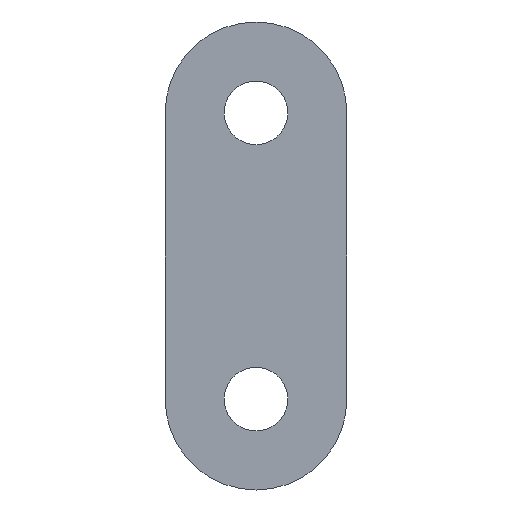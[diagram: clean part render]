
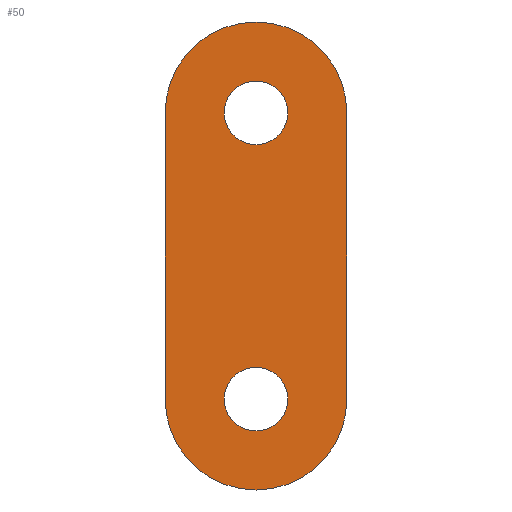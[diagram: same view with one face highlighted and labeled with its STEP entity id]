
A CAD part, left-side view. The second image highlights one B-rep face of the part: STEP entity #50.
In plain terms, the highlighted planar face has unit normal (-1, 0, 0).
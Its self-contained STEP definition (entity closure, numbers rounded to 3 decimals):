
#2 = FACE_BOUND ( 'NONE', #23, .T. ) ;
#6 = EDGE_CURVE ( 'NONE', #173, #401, #378, .T. ) ;
#10 = LINE ( 'NONE', #126, #251 ) ;
#13 = CIRCLE ( 'NONE', #390, 1.05 ) ;
#19 = ORIENTED_EDGE ( 'NONE', *, *, #31, .F. ) ;
#21 = DIRECTION ( 'NONE',  ( 0., 0., -1. ) ) ;
#22 = ORIENTED_EDGE ( 'NONE', *, *, #41, .F. ) ;
#23 = EDGE_LOOP ( 'NONE', ( #216, #328 ) ) ;
#30 = VERTEX_POINT ( 'NONE', #389 ) ;
#31 = EDGE_CURVE ( 'NONE', #175, #66, #322, .T. ) ;
#41 = EDGE_CURVE ( 'NONE', #116, #319, #157, .T. ) ;
#49 = EDGE_LOOP ( 'NONE', ( #407, #62 ) ) ;
#50 = ADVANCED_FACE ( 'NONE', ( #2, #203, #423 ), #230, .F. ) ;
#55 = ORIENTED_EDGE ( 'NONE', *, *, #72, .T. ) ;
#61 = EDGE_CURVE ( 'NONE', #319, #175, #166, .T. ) ;
#62 = ORIENTED_EDGE ( 'NONE', *, *, #90, .T. ) ;
#66 = VERTEX_POINT ( 'NONE', #195 ) ;
#72 = EDGE_CURVE ( 'NONE', #373, #66, #10, .T. ) ;
#76 = AXIS2_PLACEMENT_3D ( 'NONE', #261, #146, #21 ) ;
#90 = EDGE_CURVE ( 'NONE', #401, #173, #222, .T. ) ;
#105 = EDGE_CURVE ( 'NONE', #302, #30, #209, .T. ) ;
#109 = EDGE_LOOP ( 'NONE', ( #22, #312, #55, #19, #386 ) ) ;
#111 = EDGE_CURVE ( 'NONE', #373, #116, #217, .T. ) ;
#114 = CARTESIAN_POINT ( 'NONE',  ( 0.6, 0., 1.575 ) ) ;
#116 = VERTEX_POINT ( 'NONE', #382 ) ;
#122 = DIRECTION ( 'NONE',  ( 0., 0., 1. ) ) ;
#126 = CARTESIAN_POINT ( 'NONE',  ( 0.6, -3., 1.575 ) ) ;
#136 = DIRECTION ( 'NONE',  ( 0., 0., 1. ) ) ;
#146 = DIRECTION ( 'NONE',  ( 1., 0., 0. ) ) ;
#149 = DIRECTION ( 'NONE',  ( 0., 0., -1. ) ) ;
#154 = DIRECTION ( 'NONE',  ( 0., 0., -1. ) ) ;
#157 = LINE ( 'NONE', #321, #200 ) ;
#166 = CIRCLE ( 'NONE', #202, 3. ) ;
#170 = CARTESIAN_POINT ( 'NONE',  ( 0.6, 0., 14.026 ) ) ;
#173 = VERTEX_POINT ( 'NONE', #183 ) ;
#175 = VERTEX_POINT ( 'NONE', #170 ) ;
#178 = CARTESIAN_POINT ( 'NONE',  ( 0.6, 0., 11.026 ) ) ;
#183 = CARTESIAN_POINT ( 'NONE',  ( 0.6, 0., 2.625 ) ) ;
#190 = DIRECTION ( 'NONE',  ( 1., 0., 0. ) ) ;
#194 = EDGE_CURVE ( 'NONE', #30, #302, #13, .T. ) ;
#195 = CARTESIAN_POINT ( 'NONE',  ( 0.6, -3., 11.026 ) ) ;
#199 = DIRECTION ( 'NONE',  ( 0., 0., -1. ) ) ;
#200 = VECTOR ( 'NONE', #136, 1000. ) ;
#202 = AXIS2_PLACEMENT_3D ( 'NONE', #383, #303, #199 ) ;
#203 = FACE_BOUND ( 'NONE', #49, .T. ) ;
#209 = CIRCLE ( 'NONE', #408, 1.05 ) ;
#216 = ORIENTED_EDGE ( 'NONE', *, *, #194, .T. ) ;
#217 = CIRCLE ( 'NONE', #406, 3. ) ;
#220 = DIRECTION ( 'NONE',  ( 1., 0., 0. ) ) ;
#222 = CIRCLE ( 'NONE', #76, 1.05 ) ;
#230 = PLANE ( 'NONE',  #250 ) ;
#233 = DIRECTION ( 'NONE',  ( 0., 0., -1. ) ) ;
#239 = CARTESIAN_POINT ( 'NONE',  ( 0.6, 0., 1.575 ) ) ;
#248 = DIRECTION ( 'NONE',  ( 0., 0., -1. ) ) ;
#250 = AXIS2_PLACEMENT_3D ( 'NONE', #239, #190, #351 ) ;
#251 = VECTOR ( 'NONE', #122, 1000. ) ;
#261 = CARTESIAN_POINT ( 'NONE',  ( 0.6, 0., 1.575 ) ) ;
#276 = CARTESIAN_POINT ( 'NONE',  ( 0.6, 0., 1.575 ) ) ;
#302 = VERTEX_POINT ( 'NONE', #393 ) ;
#303 = DIRECTION ( 'NONE',  ( 1., 0., 0. ) ) ;
#312 = ORIENTED_EDGE ( 'NONE', *, *, #111, .F. ) ;
#319 = VERTEX_POINT ( 'NONE', #395 ) ;
#320 = CARTESIAN_POINT ( 'NONE',  ( 0.6, 0., 11.026 ) ) ;
#321 = CARTESIAN_POINT ( 'NONE',  ( 0.6, 3., 1.575 ) ) ;
#322 = CIRCLE ( 'NONE', #366, 3. ) ;
#328 = ORIENTED_EDGE ( 'NONE', *, *, #105, .T. ) ;
#340 = DIRECTION ( 'NONE',  ( 1., 0., 0. ) ) ;
#351 = DIRECTION ( 'NONE',  ( 0., 0., -1. ) ) ;
#366 = AXIS2_PLACEMENT_3D ( 'NONE', #178, #371, #149 ) ;
#371 = DIRECTION ( 'NONE',  ( 1., 0., 0. ) ) ;
#373 = VERTEX_POINT ( 'NONE', #381 ) ;
#376 = CARTESIAN_POINT ( 'NONE',  ( 0.6, 0., 0.525 ) ) ;
#378 = CIRCLE ( 'NONE', #394, 1.05 ) ;
#381 = CARTESIAN_POINT ( 'NONE',  ( 0.6, -3., 1.575 ) ) ;
#382 = CARTESIAN_POINT ( 'NONE',  ( 0.6, 3., 1.575 ) ) ;
#383 = CARTESIAN_POINT ( 'NONE',  ( 0.6, 0., 11.026 ) ) ;
#386 = ORIENTED_EDGE ( 'NONE', *, *, #61, .F. ) ;
#389 = CARTESIAN_POINT ( 'NONE',  ( 0.6, 0., 12.076 ) ) ;
#390 = AXIS2_PLACEMENT_3D ( 'NONE', #400, #399, #398 ) ;
#393 = CARTESIAN_POINT ( 'NONE',  ( 0.6, 0., 9.976 ) ) ;
#394 = AXIS2_PLACEMENT_3D ( 'NONE', #276, #220, #154 ) ;
#395 = CARTESIAN_POINT ( 'NONE',  ( 0.6, 3., 11.026 ) ) ;
#398 = DIRECTION ( 'NONE',  ( 0., 0., -1. ) ) ;
#399 = DIRECTION ( 'NONE',  ( 1., 0., 0. ) ) ;
#400 = CARTESIAN_POINT ( 'NONE',  ( 0.6, 0., 11.026 ) ) ;
#401 = VERTEX_POINT ( 'NONE', #376 ) ;
#406 = AXIS2_PLACEMENT_3D ( 'NONE', #114, #340, #248 ) ;
#407 = ORIENTED_EDGE ( 'NONE', *, *, #6, .T. ) ;
#408 = AXIS2_PLACEMENT_3D ( 'NONE', #320, #417, #233 ) ;
#417 = DIRECTION ( 'NONE',  ( 1., 0., 0. ) ) ;
#423 = FACE_OUTER_BOUND ( 'NONE', #109, .T. ) ;
